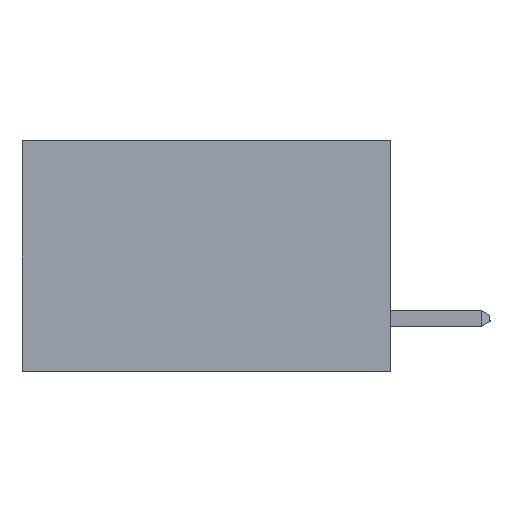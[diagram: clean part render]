
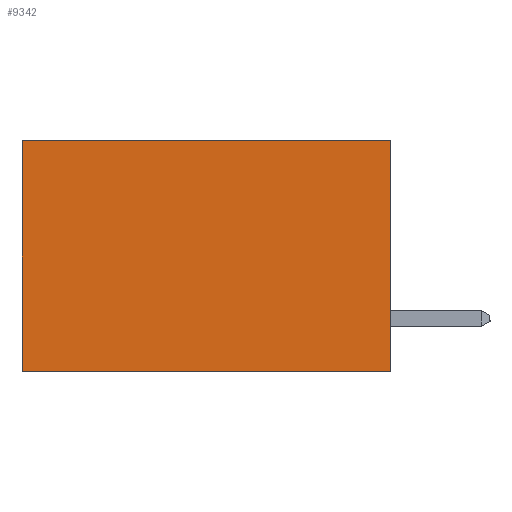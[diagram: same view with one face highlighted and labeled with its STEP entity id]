
A CAD part, left-side view. The second image highlights one B-rep face of the part: STEP entity #9342.
In plain terms, the highlighted planar face has unit normal (-1, 0, 0).
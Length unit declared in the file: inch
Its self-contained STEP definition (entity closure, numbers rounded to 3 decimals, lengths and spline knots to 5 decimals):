
#643 = VERTEX_POINT ( 'NONE', #8383 ) ;
#810 = CARTESIAN_POINT ( 'NONE',  ( 0.277, 0.59, -0.37 ) ) ;
#1055 = CARTESIAN_POINT ( 'NONE',  ( 0.277, 0., -0.37 ) ) ;
#1479 = CARTESIAN_POINT ( 'NONE',  ( 0.277, 0., -0.37 ) ) ;
#2155 = VERTEX_POINT ( 'NONE', #9685 ) ;
#2370 = VERTEX_POINT ( 'NONE', #2943 ) ;
#2532 = DIRECTION ( 'NONE',  ( 0., 0., -1. ) ) ;
#2943 = CARTESIAN_POINT ( 'NONE',  ( 0.277, 0.59, -0.37 ) ) ;
#3085 = DIRECTION ( 'NONE',  ( 0., 1., 0. ) ) ;
#3599 = LINE ( 'NONE', #810, #8739 ) ;
#4660 = VECTOR ( 'NONE', #9024, 39.37008 ) ;
#4688 = CARTESIAN_POINT ( 'NONE',  ( 0.277, 0., -0.37 ) ) ;
#4897 = EDGE_LOOP ( 'NONE', ( #5360, #10940, #9360, #6974 ) ) ;
#4958 = FACE_OUTER_BOUND ( 'NONE', #4897, .T. ) ;
#4968 = AXIS2_PLACEMENT_3D ( 'NONE', #1479, #8664, #2532 ) ;
#5360 = ORIENTED_EDGE ( 'NONE', *, *, #10781, .T. ) ;
#5994 = EDGE_CURVE ( 'NONE', #6082, #2370, #12739, .T. ) ;
#6082 = VERTEX_POINT ( 'NONE', #4688 ) ;
#6154 = VECTOR ( 'NONE', #6735, 39.37008 ) ;
#6432 = EDGE_CURVE ( 'NONE', #643, #6082, #12721, .T. ) ;
#6735 = DIRECTION ( 'NONE',  ( 0., 1., 0. ) ) ;
#6974 = ORIENTED_EDGE ( 'NONE', *, *, #12901, .T. ) ;
#7663 = PLANE ( 'NONE',  #4968 ) ;
#8383 = CARTESIAN_POINT ( 'NONE',  ( 0.277, 0., 0. ) ) ;
#8664 = DIRECTION ( 'NONE',  ( 1., 0., 0. ) ) ;
#8739 = VECTOR ( 'NONE', #10055, 39.37008 ) ;
#8849 = LINE ( 'NONE', #10826, #6154 ) ;
#8887 = CARTESIAN_POINT ( 'NONE',  ( 0.277, 0., -0.37 ) ) ;
#9024 = DIRECTION ( 'NONE',  ( 0., 0., -1. ) ) ;
#9342 = ADVANCED_FACE ( 'NONE', ( #4958 ), #7663, .F. ) ;
#9360 = ORIENTED_EDGE ( 'NONE', *, *, #6432, .F. ) ;
#9685 = CARTESIAN_POINT ( 'NONE',  ( 0.277, 0.59, 0. ) ) ;
#10055 = DIRECTION ( 'NONE',  ( 0., 0., -1. ) ) ;
#10781 = EDGE_CURVE ( 'NONE', #2155, #2370, #3599, .T. ) ;
#10826 = CARTESIAN_POINT ( 'NONE',  ( 0.277, 0., 0. ) ) ;
#10940 = ORIENTED_EDGE ( 'NONE', *, *, #5994, .F. ) ;
#12428 = VECTOR ( 'NONE', #3085, 39.37008 ) ;
#12721 = LINE ( 'NONE', #8887, #4660 ) ;
#12739 = LINE ( 'NONE', #1055, #12428 ) ;
#12901 = EDGE_CURVE ( 'NONE', #643, #2155, #8849, .T. ) ;
